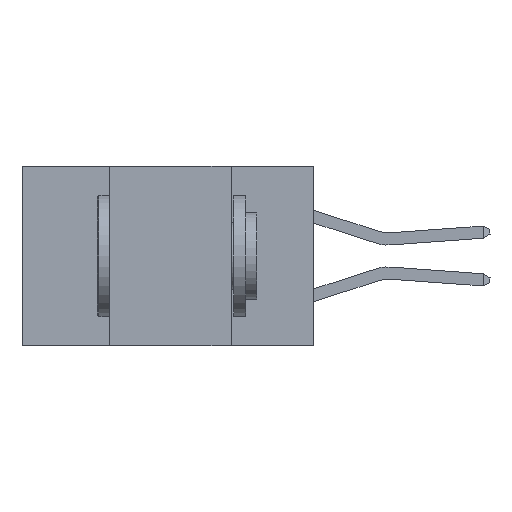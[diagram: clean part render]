
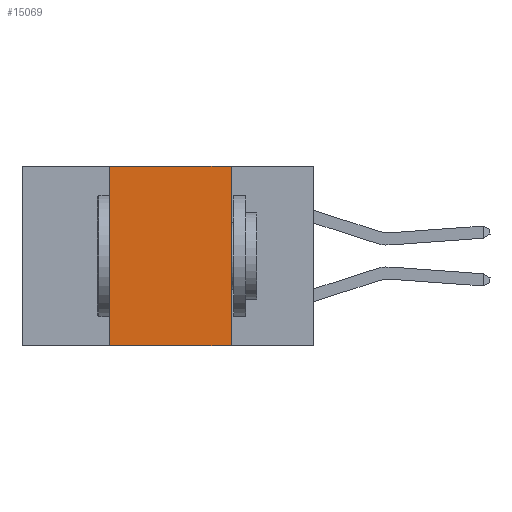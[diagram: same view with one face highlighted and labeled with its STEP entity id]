
A CAD part, left-side view. The second image highlights one B-rep face of the part: STEP entity #15069.
In plain terms, the highlighted planar face has unit normal (-1, 0, 0).
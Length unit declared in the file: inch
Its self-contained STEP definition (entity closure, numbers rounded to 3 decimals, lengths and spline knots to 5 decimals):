
#1718 = ORIENTED_EDGE ( 'NONE', *, *, #5856, .F. ) ;
#4665 = DIRECTION ( 'NONE',  ( 0., -1., 0. ) ) ;
#5187 = CARTESIAN_POINT ( 'NONE',  ( 0., 0.6, -0.37 ) ) ;
#5856 = EDGE_CURVE ( 'NONE', #20404, #19559, #21739, .T. ) ;
#5881 = DIRECTION ( 'NONE',  ( 0., -1., 0. ) ) ;
#6522 = CARTESIAN_POINT ( 'NONE',  ( 0., 0.17, -0.37 ) ) ;
#7968 = VECTOR ( 'NONE', #11902, 39.37008 ) ;
#10009 = VERTEX_POINT ( 'NONE', #6522 ) ;
#10870 = CARTESIAN_POINT ( 'NONE',  ( 0., 0.42, 0. ) ) ;
#11902 = DIRECTION ( 'NONE',  ( 0., 0., 1. ) ) ;
#12802 = ORIENTED_EDGE ( 'NONE', *, *, #13393, .F. ) ;
#13393 = EDGE_CURVE ( 'NONE', #33769, #20404, #18871, .T. ) ;
#15069 = ADVANCED_FACE ( 'NONE', ( #30060 ), #19065, .F. ) ;
#16259 = ORIENTED_EDGE ( 'NONE', *, *, #17302, .F. ) ;
#16410 = CARTESIAN_POINT ( 'NONE',  ( 0., 0.42, 0. ) ) ;
#16855 = CARTESIAN_POINT ( 'NONE',  ( 0., 0.6, 0. ) ) ;
#17302 = EDGE_CURVE ( 'NONE', #19559, #10009, #36403, .T. ) ;
#18481 = VECTOR ( 'NONE', #19141, 39.37008 ) ;
#18871 = LINE ( 'NONE', #10870, #7968 ) ;
#19065 = PLANE ( 'NONE',  #25040 ) ;
#19141 = DIRECTION ( 'NONE',  ( 0., 0., -1. ) ) ;
#19559 = VERTEX_POINT ( 'NONE', #32842 ) ;
#20404 = VERTEX_POINT ( 'NONE', #16410 ) ;
#21561 = DIRECTION ( 'NONE',  ( 0., 0., -1. ) ) ;
#21739 = LINE ( 'NONE', #16855, #24568 ) ;
#24568 = VECTOR ( 'NONE', #5881, 39.37008 ) ;
#24929 = CARTESIAN_POINT ( 'NONE',  ( 0., 0.17, 0. ) ) ;
#25040 = AXIS2_PLACEMENT_3D ( 'NONE', #27894, #36746, #21561 ) ;
#25661 = ORIENTED_EDGE ( 'NONE', *, *, #36863, .T. ) ;
#26019 = LINE ( 'NONE', #5187, #31229 ) ;
#27894 = CARTESIAN_POINT ( 'NONE',  ( 0., 0.6, 0. ) ) ;
#28303 = EDGE_LOOP ( 'NONE', ( #16259, #1718, #12802, #25661 ) ) ;
#30060 = FACE_OUTER_BOUND ( 'NONE', #28303, .T. ) ;
#31229 = VECTOR ( 'NONE', #4665, 39.37008 ) ;
#32842 = CARTESIAN_POINT ( 'NONE',  ( 0., 0.17, 0. ) ) ;
#33769 = VERTEX_POINT ( 'NONE', #33932 ) ;
#33932 = CARTESIAN_POINT ( 'NONE',  ( 0., 0.42, -0.37 ) ) ;
#36403 = LINE ( 'NONE', #24929, #18481 ) ;
#36746 = DIRECTION ( 'NONE',  ( 1., 0., 0. ) ) ;
#36863 = EDGE_CURVE ( 'NONE', #33769, #10009, #26019, .T. ) ;
